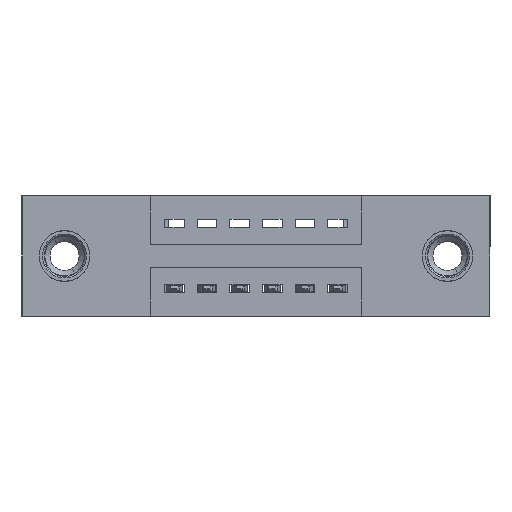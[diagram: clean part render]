
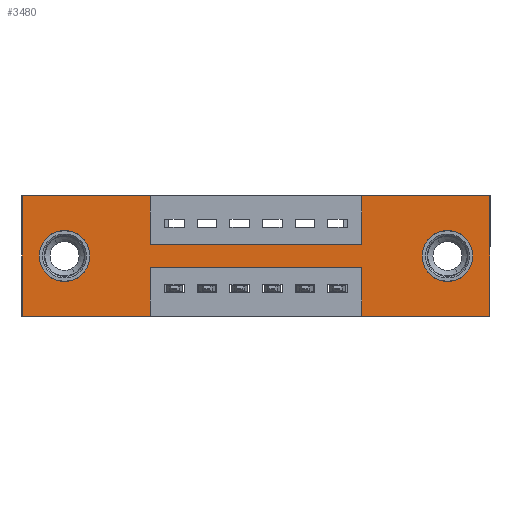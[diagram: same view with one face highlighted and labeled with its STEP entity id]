
A CAD part, front view. The second image highlights one B-rep face of the part: STEP entity #3480.
In plain terms, the highlighted planar face has unit normal (0, -1, 0).
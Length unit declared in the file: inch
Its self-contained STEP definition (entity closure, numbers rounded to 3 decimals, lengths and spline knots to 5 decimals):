
#2 = ORIENTED_EDGE ( 'NONE', *, *, #3226, .T. ) ;
#53 = CARTESIAN_POINT ( 'NONE',  ( 1.0425, 0., -0.37 ) ) ;
#289 = VECTOR ( 'NONE', #655, 39.37008 ) ;
#311 = DIRECTION ( 'NONE',  ( 0., 1., 0. ) ) ;
#409 = ORIENTED_EDGE ( 'NONE', *, *, #4704, .T. ) ;
#431 = CARTESIAN_POINT ( 'NONE',  ( 0.3925, 0., 0. ) ) ;
#497 = VERTEX_POINT ( 'NONE', #13565 ) ;
#593 = LINE ( 'NONE', #1377, #11930 ) ;
#655 = DIRECTION ( 'NONE',  ( 1., 0., 0. ) ) ;
#682 = ORIENTED_EDGE ( 'NONE', *, *, #6743, .F. ) ;
#1030 = EDGE_CURVE ( 'NONE', #10214, #497, #3713, .T. ) ;
#1339 = DIRECTION ( 'NONE',  ( 0., 0., -1. ) ) ;
#1347 = VECTOR ( 'NONE', #12376, 39.37008 ) ;
#1377 = CARTESIAN_POINT ( 'NONE',  ( 0.3925, 0., -0.37 ) ) ;
#1437 = EDGE_CURVE ( 'NONE', #6000, #6574, #8588, .T. ) ;
#1525 = VERTEX_POINT ( 'NONE', #9420 ) ;
#1754 = EDGE_CURVE ( 'NONE', #6916, #11319, #9525, .T. ) ;
#1922 = DIRECTION ( 'NONE',  ( 0., 0., 1. ) ) ;
#2016 = DIRECTION ( 'NONE',  ( 0., 1., 0. ) ) ;
#2087 = CARTESIAN_POINT ( 'NONE',  ( 0.3925, 0., -0.15 ) ) ;
#2125 = DIRECTION ( 'NONE',  ( 0., 1., 0. ) ) ;
#2414 = ORIENTED_EDGE ( 'NONE', *, *, #5436, .F. ) ;
#2459 = DIRECTION ( 'NONE',  ( 0., 0., 1. ) ) ;
#2698 = ORIENTED_EDGE ( 'NONE', *, *, #10327, .F. ) ;
#2708 = CARTESIAN_POINT ( 'NONE',  ( 0., 0., 0. ) ) ;
#2753 = CIRCLE ( 'NONE', #9308, 0.078 ) ;
#2754 = CARTESIAN_POINT ( 'NONE',  ( 0., 0., 0. ) ) ;
#3100 = CARTESIAN_POINT ( 'NONE',  ( 1.0425, 0., 0. ) ) ;
#3226 = EDGE_CURVE ( 'NONE', #1525, #10974, #7916, .T. ) ;
#3249 = CARTESIAN_POINT ( 'NONE',  ( 1.305, 0., -0.185 ) ) ;
#3389 = CARTESIAN_POINT ( 'NONE',  ( 1.435, 0., -0.37 ) ) ;
#3448 = CARTESIAN_POINT ( 'NONE',  ( 0.13, 0., -0.185 ) ) ;
#3451 = ORIENTED_EDGE ( 'NONE', *, *, #1754, .F. ) ;
#3470 = VERTEX_POINT ( 'NONE', #12429 ) ;
#3480 = ADVANCED_FACE ( 'NONE', ( #5305, #13963, #10676 ), #8237, .T. ) ;
#3515 = VERTEX_POINT ( 'NONE', #6035 ) ;
#3556 = LINE ( 'NONE', #53, #10117 ) ;
#3713 = LINE ( 'NONE', #7176, #9943 ) ;
#3722 = ORIENTED_EDGE ( 'NONE', *, *, #11573, .F. ) ;
#3746 = DIRECTION ( 'NONE',  ( 0., -1., 0. ) ) ;
#3976 = LINE ( 'NONE', #2754, #289 ) ;
#4286 = AXIS2_PLACEMENT_3D ( 'NONE', #7112, #3746, #13513 ) ;
#4293 = DIRECTION ( 'NONE',  ( 0., 0., -1. ) ) ;
#4347 = DIRECTION ( 'NONE',  ( 0., 0., 1. ) ) ;
#4704 = EDGE_CURVE ( 'NONE', #10974, #1525, #9794, .T. ) ;
#4706 = VERTEX_POINT ( 'NONE', #2087 ) ;
#4768 = DIRECTION ( 'NONE',  ( 1., 0., 0. ) ) ;
#4787 = VERTEX_POINT ( 'NONE', #3389 ) ;
#4856 = CARTESIAN_POINT ( 'NONE',  ( 1.435, 0., 0. ) ) ;
#5305 = FACE_BOUND ( 'NONE', #5823, .T. ) ;
#5373 = LINE ( 'NONE', #8701, #5563 ) ;
#5436 = EDGE_CURVE ( 'NONE', #4706, #12562, #11517, .T. ) ;
#5563 = VECTOR ( 'NONE', #1339, 39.37008 ) ;
#5777 = LINE ( 'NONE', #8571, #13915 ) ;
#5823 = EDGE_LOOP ( 'NONE', ( #2, #409 ) ) ;
#5832 = EDGE_CURVE ( 'NONE', #6574, #4787, #5777, .T. ) ;
#6000 = VERTEX_POINT ( 'NONE', #12028 ) ;
#6035 = CARTESIAN_POINT ( 'NONE',  ( 0.13, 0., -0.263 ) ) ;
#6280 = DIRECTION ( 'NONE',  ( 0., 0., -1. ) ) ;
#6552 = EDGE_LOOP ( 'NONE', ( #10407, #12734 ) ) ;
#6574 = VERTEX_POINT ( 'NONE', #4856 ) ;
#6677 = VECTOR ( 'NONE', #4768, 39.37008 ) ;
#6727 = LINE ( 'NONE', #2708, #12086 ) ;
#6743 = EDGE_CURVE ( 'NONE', #12562, #6000, #7515, .T. ) ;
#6916 = VERTEX_POINT ( 'NONE', #10679 ) ;
#7112 = CARTESIAN_POINT ( 'NONE',  ( 0., 0., -0.37 ) ) ;
#7176 = CARTESIAN_POINT ( 'NONE',  ( 0., 0., -0.37 ) ) ;
#7195 = CARTESIAN_POINT ( 'NONE',  ( 0.3925, 0., -0.37 ) ) ;
#7270 = CARTESIAN_POINT ( 'NONE',  ( 0., 0., -0.37 ) ) ;
#7515 = LINE ( 'NONE', #3100, #12685 ) ;
#7573 = EDGE_CURVE ( 'NONE', #3515, #9262, #11646, .T. ) ;
#7606 = ORIENTED_EDGE ( 'NONE', *, *, #5832, .F. ) ;
#7807 = ORIENTED_EDGE ( 'NONE', *, *, #11838, .F. ) ;
#7916 = CIRCLE ( 'NONE', #9043, 0.078 ) ;
#7928 = EDGE_CURVE ( 'NONE', #11731, #11072, #3976, .T. ) ;
#8135 = LINE ( 'NONE', #7270, #10357 ) ;
#8182 = DIRECTION ( 'NONE',  ( 0., 0., 1. ) ) ;
#8237 = PLANE ( 'NONE',  #4286 ) ;
#8260 = EDGE_CURVE ( 'NONE', #11072, #4706, #5373, .T. ) ;
#8299 = DIRECTION ( 'NONE',  ( -1., 0., 0. ) ) ;
#8571 = CARTESIAN_POINT ( 'NONE',  ( 1.435, 0., 0. ) ) ;
#8588 = LINE ( 'NONE', #13511, #1347 ) ;
#8670 = ORIENTED_EDGE ( 'NONE', *, *, #12053, .F. ) ;
#8701 = CARTESIAN_POINT ( 'NONE',  ( 0.3925, 0., 0. ) ) ;
#8871 = CARTESIAN_POINT ( 'NONE',  ( 1.0425, 0., -0.15 ) ) ;
#9043 = AXIS2_PLACEMENT_3D ( 'NONE', #10674, #11810, #6280 ) ;
#9262 = VERTEX_POINT ( 'NONE', #13743 ) ;
#9308 = AXIS2_PLACEMENT_3D ( 'NONE', #3448, #311, #2459 ) ;
#9378 = ORIENTED_EDGE ( 'NONE', *, *, #7928, .F. ) ;
#9420 = CARTESIAN_POINT ( 'NONE',  ( 1.305, 0., -0.107 ) ) ;
#9439 = DIRECTION ( 'NONE',  ( -1., 0., 0. ) ) ;
#9489 = ORIENTED_EDGE ( 'NONE', *, *, #1030, .F. ) ;
#9525 = LINE ( 'NONE', #9734, #10728 ) ;
#9734 = CARTESIAN_POINT ( 'NONE',  ( 0.3925, 0., -0.22 ) ) ;
#9794 = CIRCLE ( 'NONE', #10144, 0.078 ) ;
#9868 = EDGE_CURVE ( 'NONE', #9262, #3515, #2753, .T. ) ;
#9943 = VECTOR ( 'NONE', #9439, 39.37008 ) ;
#10047 = ORIENTED_EDGE ( 'NONE', *, *, #1437, .F. ) ;
#10117 = VECTOR ( 'NONE', #4347, 39.37008 ) ;
#10144 = AXIS2_PLACEMENT_3D ( 'NONE', #3249, #2125, #4293 ) ;
#10214 = VERTEX_POINT ( 'NONE', #7195 ) ;
#10248 = CARTESIAN_POINT ( 'NONE',  ( 0., 0., 0. ) ) ;
#10327 = EDGE_CURVE ( 'NONE', #3470, #6916, #3556, .T. ) ;
#10357 = VECTOR ( 'NONE', #8299, 39.37008 ) ;
#10407 = ORIENTED_EDGE ( 'NONE', *, *, #9868, .T. ) ;
#10674 = CARTESIAN_POINT ( 'NONE',  ( 1.305, 0., -0.185 ) ) ;
#10676 = FACE_OUTER_BOUND ( 'NONE', #11265, .T. ) ;
#10679 = CARTESIAN_POINT ( 'NONE',  ( 1.0425, 0., -0.22 ) ) ;
#10728 = VECTOR ( 'NONE', #11887, 39.37008 ) ;
#10732 = CARTESIAN_POINT ( 'NONE',  ( 0.13, 0., -0.185 ) ) ;
#10974 = VERTEX_POINT ( 'NONE', #11207 ) ;
#11072 = VERTEX_POINT ( 'NONE', #431 ) ;
#11207 = CARTESIAN_POINT ( 'NONE',  ( 1.305, 0., -0.263 ) ) ;
#11265 = EDGE_LOOP ( 'NONE', ( #3722, #3451, #2698, #7807, #7606, #10047, #682, #2414, #13791, #9378, #8670, #9489 ) ) ;
#11319 = VERTEX_POINT ( 'NONE', #13354 ) ;
#11407 = CARTESIAN_POINT ( 'NONE',  ( 0.3925, 0., -0.15 ) ) ;
#11517 = LINE ( 'NONE', #11407, #6677 ) ;
#11573 = EDGE_CURVE ( 'NONE', #11319, #10214, #593, .T. ) ;
#11646 = CIRCLE ( 'NONE', #13337, 0.078 ) ;
#11731 = VERTEX_POINT ( 'NONE', #10248 ) ;
#11810 = DIRECTION ( 'NONE',  ( 0., 1., 0. ) ) ;
#11838 = EDGE_CURVE ( 'NONE', #4787, #3470, #8135, .T. ) ;
#11887 = DIRECTION ( 'NONE',  ( -1., 0., 0. ) ) ;
#11930 = VECTOR ( 'NONE', #13293, 39.37008 ) ;
#11970 = DIRECTION ( 'NONE',  ( 0., 0., 1. ) ) ;
#12028 = CARTESIAN_POINT ( 'NONE',  ( 1.0425, 0., 0. ) ) ;
#12053 = EDGE_CURVE ( 'NONE', #497, #11731, #6727, .T. ) ;
#12086 = VECTOR ( 'NONE', #8182, 39.37008 ) ;
#12376 = DIRECTION ( 'NONE',  ( 1., 0., 0. ) ) ;
#12429 = CARTESIAN_POINT ( 'NONE',  ( 1.0425, 0., -0.37 ) ) ;
#12562 = VERTEX_POINT ( 'NONE', #8871 ) ;
#12685 = VECTOR ( 'NONE', #11970, 39.37008 ) ;
#12734 = ORIENTED_EDGE ( 'NONE', *, *, #7573, .T. ) ;
#13061 = DIRECTION ( 'NONE',  ( 0., 0., -1. ) ) ;
#13293 = DIRECTION ( 'NONE',  ( 0., 0., -1. ) ) ;
#13337 = AXIS2_PLACEMENT_3D ( 'NONE', #10732, #2016, #1922 ) ;
#13354 = CARTESIAN_POINT ( 'NONE',  ( 0.3925, 0., -0.22 ) ) ;
#13511 = CARTESIAN_POINT ( 'NONE',  ( 0., 0., 0. ) ) ;
#13513 = DIRECTION ( 'NONE',  ( 0., 0., -1. ) ) ;
#13565 = CARTESIAN_POINT ( 'NONE',  ( 0., 0., -0.37 ) ) ;
#13743 = CARTESIAN_POINT ( 'NONE',  ( 0.13, 0., -0.107 ) ) ;
#13791 = ORIENTED_EDGE ( 'NONE', *, *, #8260, .F. ) ;
#13915 = VECTOR ( 'NONE', #13061, 39.37008 ) ;
#13963 = FACE_BOUND ( 'NONE', #6552, .T. ) ;
